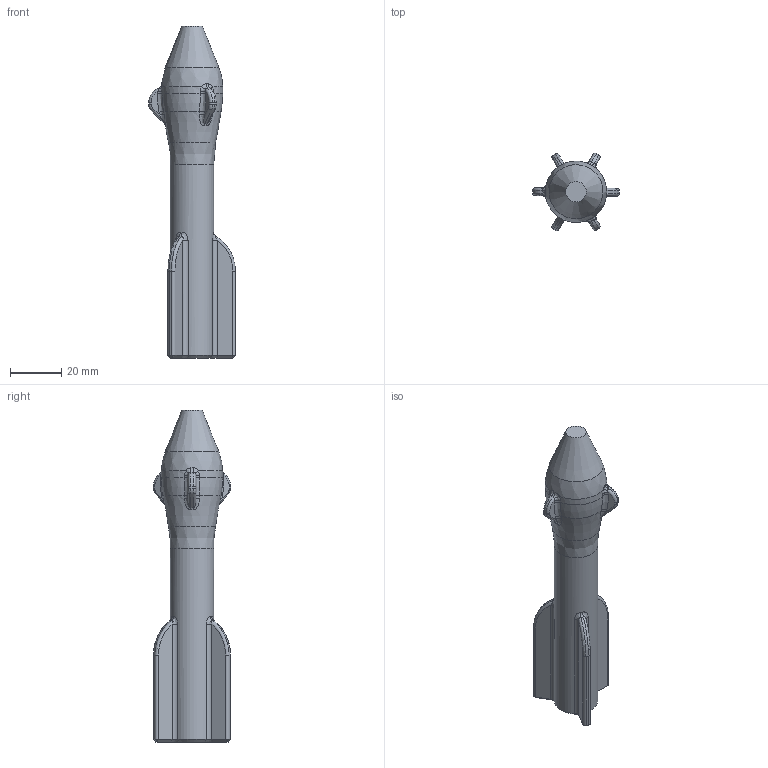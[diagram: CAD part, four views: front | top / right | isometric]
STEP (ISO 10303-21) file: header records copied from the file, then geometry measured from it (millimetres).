
FILE_DESCRIPTION(('FreeCAD Model'),'2;1');
FILE_NAME('Open CASCADE Shape Model','2022-10-05T16:42:57',('Author'),( ''),'Open CASCADE STEP processor 7.6','FreeCAD','Unknown');
FILE_SCHEMA(('AUTOMOTIVE_DESIGN { 1 0 10303 214 1 1 1 1 }'));
Length unit declared in the file: millimetre
Products named in the file (1): Body
Bounding box: 34 x 30.21 x 130 mm (x, y, z)
Volume: 30458.3 mm3; surface area: 12829.1 mm2
Topology: 1 solids, 1 shells, 165 faces, 379 edges, 211 vertices
Faces by surface type: bspline 51, cylinder 44, plane 33, cone 19, torus 18
Full cylindrical faces by diameter (mm): 10 x1, 17 x1
Entity records: 22027 total; most frequent: CARTESIAN_POINT 15541, DIRECTION 962, ORIENTED_EDGE 746, PCURVE 746, DEFINITIONAL_REPRESENTATION 746, LINE 521, VECTOR 521, EDGE_CURVE 373
